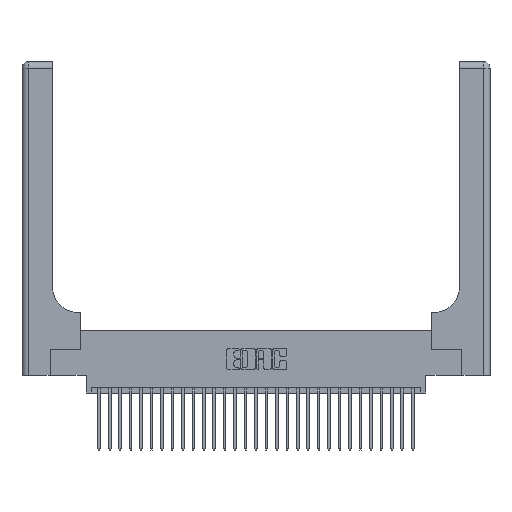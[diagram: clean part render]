
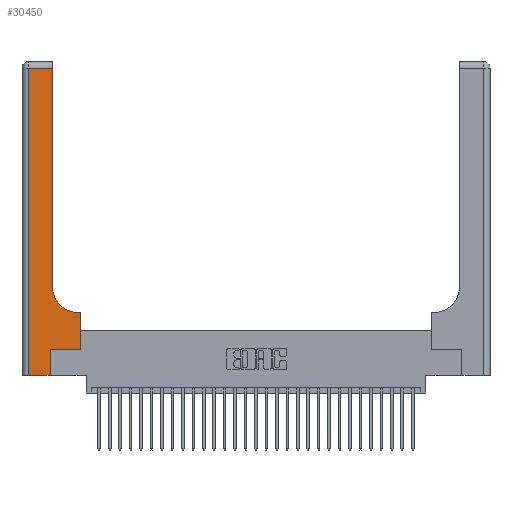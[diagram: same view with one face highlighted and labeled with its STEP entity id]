
A CAD part, top view. The second image highlights one B-rep face of the part: STEP entity #30450.
In plain terms, the highlighted planar face has unit normal (0, 0, 1).
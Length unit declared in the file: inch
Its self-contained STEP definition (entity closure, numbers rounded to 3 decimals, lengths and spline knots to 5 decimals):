
#319 = VERTEX_POINT ( 'NONE', #22022 ) ;
#637 = CARTESIAN_POINT ( 'NONE',  ( 0.5585, 0.25, 0.37 ) ) ;
#790 = EDGE_CURVE ( 'NONE', #17839, #26868, #15879, .T. ) ;
#1018 = ORIENTED_EDGE ( 'NONE', *, *, #29801, .T. ) ;
#1354 = DIRECTION ( 'NONE',  ( -1., 0., 0. ) ) ;
#1907 = VERTEX_POINT ( 'NONE', #8115 ) ;
#2967 = CARTESIAN_POINT ( 'NONE',  ( 0.5585, 0.6, 0.37 ) ) ;
#3104 = DIRECTION ( 'NONE',  ( 0., 1., 0. ) ) ;
#3594 = CARTESIAN_POINT ( 'NONE',  ( 0.06, 3., 0.37 ) ) ;
#4163 = LINE ( 'NONE', #7193, #9067 ) ;
#4227 = DIRECTION ( 'NONE',  ( 0., 0., -1. ) ) ;
#4449 = VERTEX_POINT ( 'NONE', #17795 ) ;
#5366 = CARTESIAN_POINT ( 'NONE',  ( 0.2915, 0.6, 0.37 ) ) ;
#5463 = CARTESIAN_POINT ( 'NONE',  ( 0.2915, 3., 0.37 ) ) ;
#5621 = DIRECTION ( 'NONE',  ( 0., 0., -1. ) ) ;
#5944 = VECTOR ( 'NONE', #24691, 39.37008 ) ;
#6674 = ORIENTED_EDGE ( 'NONE', *, *, #19701, .T. ) ;
#6727 = LINE ( 'NONE', #5366, #5944 ) ;
#7193 = CARTESIAN_POINT ( 'NONE',  ( 0.269, 0., 0.37 ) ) ;
#7626 = DIRECTION ( 'NONE',  ( 1., 0., 0. ) ) ;
#7801 = ORIENTED_EDGE ( 'NONE', *, *, #30613, .T. ) ;
#7889 = DIRECTION ( 'NONE',  ( 0., 1., 0. ) ) ;
#8105 = FACE_OUTER_BOUND ( 'NONE', #9914, .T. ) ;
#8115 = CARTESIAN_POINT ( 'NONE',  ( 0.06, 2.94, 0.37 ) ) ;
#8443 = ORIENTED_EDGE ( 'NONE', *, *, #23976, .T. ) ;
#9067 = VECTOR ( 'NONE', #9592, 39.37008 ) ;
#9592 = DIRECTION ( 'NONE',  ( 0., 1., 0. ) ) ;
#9914 = EDGE_LOOP ( 'NONE', ( #22338, #24956, #15849, #6674, #10384, #14324, #1018, #8443, #7801 ) ) ;
#10077 = EDGE_CURVE ( 'NONE', #1907, #23453, #25865, .T. ) ;
#10384 = ORIENTED_EDGE ( 'NONE', *, *, #28966, .T. ) ;
#11261 = VECTOR ( 'NONE', #3104, 39.37008 ) ;
#11677 = EDGE_CURVE ( 'NONE', #11834, #1907, #25236, .T. ) ;
#11834 = VERTEX_POINT ( 'NONE', #28488 ) ;
#12661 = VERTEX_POINT ( 'NONE', #24387 ) ;
#13872 = VERTEX_POINT ( 'NONE', #2967 ) ;
#14324 = ORIENTED_EDGE ( 'NONE', *, *, #790, .T. ) ;
#15157 = CARTESIAN_POINT ( 'NONE',  ( 0.269, 0.25, 0.37 ) ) ;
#15263 = DIRECTION ( 'NONE',  ( 1., 0., 0. ) ) ;
#15849 = ORIENTED_EDGE ( 'NONE', *, *, #10077, .T. ) ;
#15879 = LINE ( 'NONE', #15157, #27915 ) ;
#15883 = CARTESIAN_POINT ( 'NONE',  ( 0., 2.94, 0.37 ) ) ;
#16035 = VECTOR ( 'NONE', #7889, 39.37008 ) ;
#16412 = CIRCLE ( 'NONE', #21952, 0.25 ) ;
#17089 = AXIS2_PLACEMENT_3D ( 'NONE', #20109, #5621, #22515 ) ;
#17347 = CARTESIAN_POINT ( 'NONE',  ( 0.269, 0.25, 0.37 ) ) ;
#17795 = CARTESIAN_POINT ( 'NONE',  ( 0.2915, 0.85, 0.37 ) ) ;
#17839 = VERTEX_POINT ( 'NONE', #17347 ) ;
#18697 = VECTOR ( 'NONE', #22841, 39.37008 ) ;
#18722 = CARTESIAN_POINT ( 'NONE',  ( 0.5415, 0.85, 0.37 ) ) ;
#18837 = VECTOR ( 'NONE', #1354, 39.37008 ) ;
#19701 = EDGE_CURVE ( 'NONE', #23453, #12661, #19858, .T. ) ;
#19858 = LINE ( 'NONE', #26930, #25474 ) ;
#20109 = CARTESIAN_POINT ( 'NONE',  ( 0., 3., 0.37 ) ) ;
#21147 = DIRECTION ( 'NONE',  ( 1., 0., 0. ) ) ;
#21952 = AXIS2_PLACEMENT_3D ( 'NONE', #18722, #4227, #21147 ) ;
#22022 = CARTESIAN_POINT ( 'NONE',  ( 0.5415, 0.6, 0.37 ) ) ;
#22338 = ORIENTED_EDGE ( 'NONE', *, *, #26963, .T. ) ;
#22515 = DIRECTION ( 'NONE',  ( -1., 0., 0. ) ) ;
#22841 = DIRECTION ( 'NONE',  ( 0., -1., 0. ) ) ;
#23453 = VERTEX_POINT ( 'NONE', #29468 ) ;
#23976 = EDGE_CURVE ( 'NONE', #13872, #319, #6727, .T. ) ;
#24154 = LINE ( 'NONE', #637, #11261 ) ;
#24378 = CARTESIAN_POINT ( 'NONE',  ( 0.5585, 0.25, 0.37 ) ) ;
#24387 = CARTESIAN_POINT ( 'NONE',  ( 0.269, 0., 0.37 ) ) ;
#24691 = DIRECTION ( 'NONE',  ( -1., 0., 0. ) ) ;
#24956 = ORIENTED_EDGE ( 'NONE', *, *, #11677, .T. ) ;
#25236 = LINE ( 'NONE', #15883, #18837 ) ;
#25474 = VECTOR ( 'NONE', #7626, 39.37008 ) ;
#25865 = LINE ( 'NONE', #3594, #18697 ) ;
#26868 = VERTEX_POINT ( 'NONE', #24378 ) ;
#26930 = CARTESIAN_POINT ( 'NONE',  ( 0., 0., 0.37 ) ) ;
#26963 = EDGE_CURVE ( 'NONE', #4449, #11834, #29514, .T. ) ;
#27915 = VECTOR ( 'NONE', #15263, 39.37008 ) ;
#28488 = CARTESIAN_POINT ( 'NONE',  ( 0.2915, 2.94, 0.37 ) ) ;
#28966 = EDGE_CURVE ( 'NONE', #12661, #17839, #4163, .T. ) ;
#29468 = CARTESIAN_POINT ( 'NONE',  ( 0.06, 0., 0.37 ) ) ;
#29514 = LINE ( 'NONE', #5463, #16035 ) ;
#29572 = PLANE ( 'NONE',  #17089 ) ;
#29801 = EDGE_CURVE ( 'NONE', #26868, #13872, #24154, .T. ) ;
#30450 = ADVANCED_FACE ( 'NONE', ( #8105 ), #29572, .F. ) ;
#30613 = EDGE_CURVE ( 'NONE', #319, #4449, #16412, .T. ) ;
